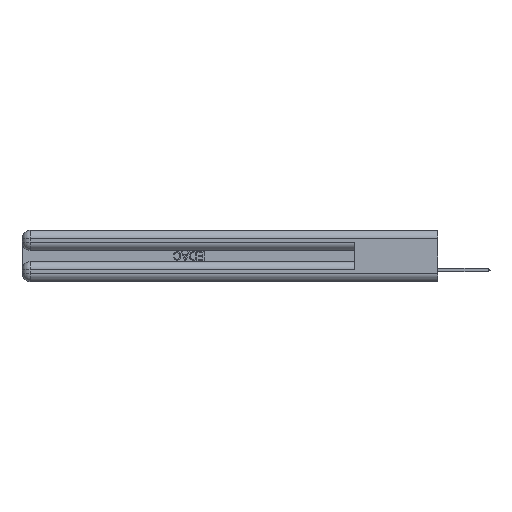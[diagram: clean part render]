
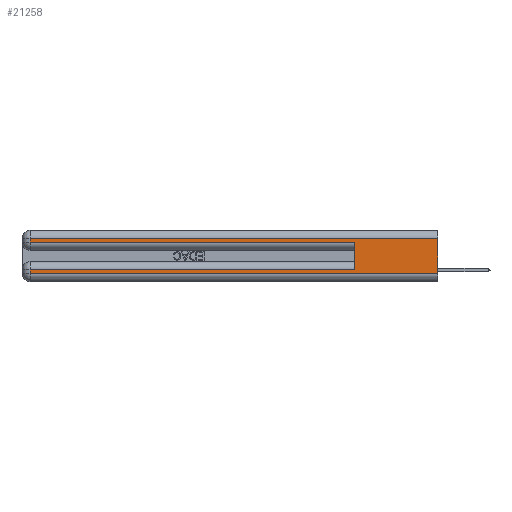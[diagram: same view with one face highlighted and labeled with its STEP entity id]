
A CAD part, left-side view. The second image highlights one B-rep face of the part: STEP entity #21258.
In plain terms, the highlighted planar face has unit normal (-1, 0, 0).
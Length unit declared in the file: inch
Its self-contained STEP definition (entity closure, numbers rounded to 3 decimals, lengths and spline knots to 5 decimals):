
#551 = VERTEX_POINT ( 'NONE', #41013 ) ;
#1147 = DIRECTION ( 'NONE',  ( 0., 0., -1. ) ) ;
#1499 = CARTESIAN_POINT ( 'NONE',  ( 0., 2.94, 0.31 ) ) ;
#2003 = VECTOR ( 'NONE', #34873, 39.37008 ) ;
#2684 = CARTESIAN_POINT ( 'NONE',  ( 0., 0., 0.37 ) ) ;
#2985 = CARTESIAN_POINT ( 'NONE',  ( 0., 2.94, 0.37 ) ) ;
#3120 = ORIENTED_EDGE ( 'NONE', *, *, #17233, .T. ) ;
#3358 = LINE ( 'NONE', #23792, #41486 ) ;
#3731 = DIRECTION ( 'NONE',  ( 0., 0., -1. ) ) ;
#3890 = VECTOR ( 'NONE', #24674, 39.37008 ) ;
#4804 = CARTESIAN_POINT ( 'NONE',  ( 0., 0., 0.31 ) ) ;
#6097 = VERTEX_POINT ( 'NONE', #46058 ) ;
#8071 = EDGE_CURVE ( 'NONE', #551, #36324, #9694, .T. ) ;
#8130 = CARTESIAN_POINT ( 'NONE',  ( 0., 0., 0.06 ) ) ;
#8468 = CARTESIAN_POINT ( 'NONE',  ( 0., 0., 0.06 ) ) ;
#8614 = AXIS2_PLACEMENT_3D ( 'NONE', #17961, #25563, #1147 ) ;
#9694 = LINE ( 'NONE', #46701, #3890 ) ;
#9744 = VECTOR ( 'NONE', #31039, 39.37008 ) ;
#11782 = ORIENTED_EDGE ( 'NONE', *, *, #17522, .T. ) ;
#13505 = CARTESIAN_POINT ( 'NONE',  ( 0., 2.94, 0.06 ) ) ;
#15618 = VECTOR ( 'NONE', #30671, 39.37008 ) ;
#16299 = CARTESIAN_POINT ( 'NONE',  ( 0., 2.94, 0.085 ) ) ;
#17233 = EDGE_CURVE ( 'NONE', #29610, #33985, #27115, .T. ) ;
#17306 = VERTEX_POINT ( 'NONE', #13505 ) ;
#17369 = VECTOR ( 'NONE', #18355, 39.37008 ) ;
#17522 = EDGE_CURVE ( 'NONE', #33985, #35936, #3358, .T. ) ;
#17961 = CARTESIAN_POINT ( 'NONE',  ( 0., 0., 0.37 ) ) ;
#18355 = DIRECTION ( 'NONE',  ( 0., 0., 1. ) ) ;
#18681 = FACE_OUTER_BOUND ( 'NONE', #19281, .T. ) ;
#19195 = VECTOR ( 'NONE', #3731, 39.37008 ) ;
#19281 = EDGE_LOOP ( 'NONE', ( #33969, #3120, #11782, #22035, #20995, #27675, #41477, #20516 ) ) ;
#20241 = CARTESIAN_POINT ( 'NONE',  ( 0., 2.94, 0.285 ) ) ;
#20516 = ORIENTED_EDGE ( 'NONE', *, *, #35072, .T. ) ;
#20995 = ORIENTED_EDGE ( 'NONE', *, *, #30553, .F. ) ;
#21239 = PLANE ( 'NONE',  #8614 ) ;
#21258 = ADVANCED_FACE ( 'NONE', ( #18681 ), #21239, .F. ) ;
#22035 = ORIENTED_EDGE ( 'NONE', *, *, #28327, .T. ) ;
#22637 = LINE ( 'NONE', #2684, #42339 ) ;
#23792 = CARTESIAN_POINT ( 'NONE',  ( 0., 2.94, 0.37 ) ) ;
#24674 = DIRECTION ( 'NONE',  ( 0., 1., 0. ) ) ;
#25563 = DIRECTION ( 'NONE',  ( 1., 0., 0. ) ) ;
#27016 = DIRECTION ( 'NONE',  ( 0., 0., -1. ) ) ;
#27115 = LINE ( 'NONE', #4804, #9744 ) ;
#27675 = ORIENTED_EDGE ( 'NONE', *, *, #8071, .T. ) ;
#27871 = LINE ( 'NONE', #8468, #15618 ) ;
#28327 = EDGE_CURVE ( 'NONE', #35936, #6097, #43028, .T. ) ;
#29610 = VERTEX_POINT ( 'NONE', #37429 ) ;
#29659 = EDGE_CURVE ( 'NONE', #29610, #32902, #22637, .T. ) ;
#30553 = EDGE_CURVE ( 'NONE', #551, #6097, #38182, .T. ) ;
#30671 = DIRECTION ( 'NONE',  ( 0., -1., 0. ) ) ;
#31039 = DIRECTION ( 'NONE',  ( 0., 1., 0. ) ) ;
#32902 = VERTEX_POINT ( 'NONE', #8130 ) ;
#33122 = EDGE_CURVE ( 'NONE', #36324, #17306, #36597, .T. ) ;
#33969 = ORIENTED_EDGE ( 'NONE', *, *, #29659, .F. ) ;
#33985 = VERTEX_POINT ( 'NONE', #1499 ) ;
#34374 = CARTESIAN_POINT ( 'NONE',  ( 0., 0., 0.285 ) ) ;
#34873 = DIRECTION ( 'NONE',  ( 0., -1., 0. ) ) ;
#35072 = EDGE_CURVE ( 'NONE', #17306, #32902, #27871, .T. ) ;
#35936 = VERTEX_POINT ( 'NONE', #20241 ) ;
#36324 = VERTEX_POINT ( 'NONE', #16299 ) ;
#36597 = LINE ( 'NONE', #2985, #19195 ) ;
#37429 = CARTESIAN_POINT ( 'NONE',  ( 0., 0., 0.31 ) ) ;
#38182 = LINE ( 'NONE', #44405, #17369 ) ;
#41013 = CARTESIAN_POINT ( 'NONE',  ( 0., 0.6, 0.085 ) ) ;
#41477 = ORIENTED_EDGE ( 'NONE', *, *, #33122, .T. ) ;
#41486 = VECTOR ( 'NONE', #27016, 39.37008 ) ;
#42339 = VECTOR ( 'NONE', #42751, 39.37008 ) ;
#42751 = DIRECTION ( 'NONE',  ( 0., 0., -1. ) ) ;
#43028 = LINE ( 'NONE', #34374, #2003 ) ;
#44405 = CARTESIAN_POINT ( 'NONE',  ( 0., 0.6, 0.145 ) ) ;
#46058 = CARTESIAN_POINT ( 'NONE',  ( 0., 0.6, 0.285 ) ) ;
#46701 = CARTESIAN_POINT ( 'NONE',  ( 0., 0., 0.085 ) ) ;
